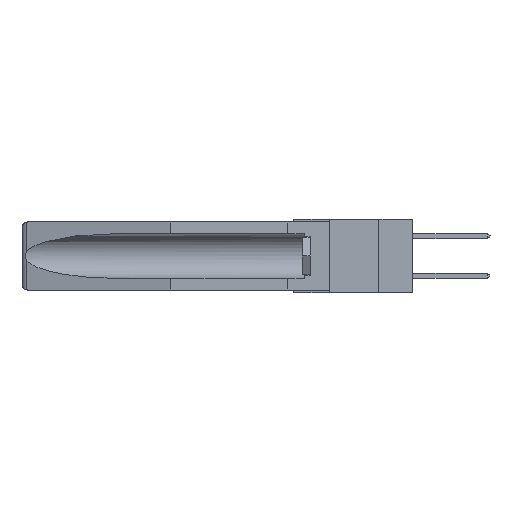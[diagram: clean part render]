
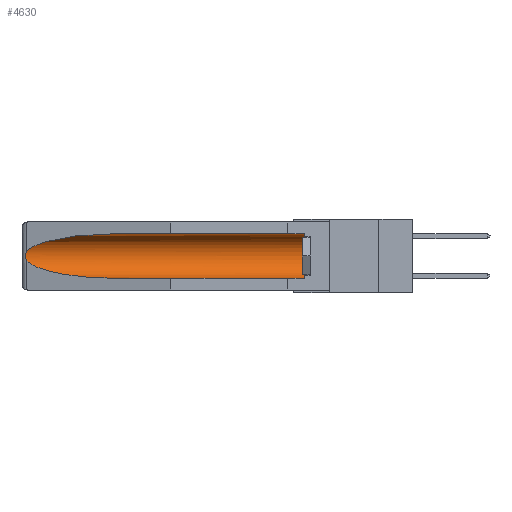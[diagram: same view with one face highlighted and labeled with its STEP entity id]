
A CAD part, left-side view. The second image highlights one B-rep face of the part: STEP entity #4630.
In plain terms, the highlighted cylindrical face has radius 2.857 mm (diameter 5.715 mm), a partial arc.
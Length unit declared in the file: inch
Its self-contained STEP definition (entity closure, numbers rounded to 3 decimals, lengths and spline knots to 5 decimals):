
#781 = CARTESIAN_POINT ( 'NONE',  ( 0.155, 1.07973, -0.284 ) ) ;
#1403 = CIRCLE ( 'NONE', #14783, 0.1125 ) ;
#1441 = CARTESIAN_POINT ( 'NONE',  ( 0.155, 0.126, -0.284 ) ) ;
#1802 = ORIENTED_EDGE ( 'NONE', *, *, #2086, .T. ) ;
#1818 = FACE_OUTER_BOUND ( 'NONE', #15287, .T. ) ;
#2026 = CARTESIAN_POINT ( 'NONE',  ( 0.155, -0.30754, -0.284 ) ) ;
#2086 = EDGE_CURVE ( 'NONE', #15935, #18991, #5848, .T. ) ;
#2349 = CARTESIAN_POINT ( 'NONE',  ( 0.2675, 1.53308, -0.17534 ) ) ;
#2480 = EDGE_CURVE ( 'NONE', #6593, #8802, #5024, .T. ) ;
#2681 = AXIS2_PLACEMENT_3D ( 'NONE', #6621, #21025, #12942 ) ;
#3083 = ORIENTED_EDGE ( 'NONE', *, *, #21367, .T. ) ;
#3285 = EDGE_CURVE ( 'NONE', #18991, #6593, #23365, .T. ) ;
#4249 = CARTESIAN_POINT ( 'NONE',  ( 0.21114, 1.30732, -0.059 ) ) ;
#4428 = CARTESIAN_POINT ( 'NONE',  ( 0.26655, 1.53094, -0.18657 ) ) ;
#4630 = ADVANCED_FACE ( 'NONE', ( #1818 ), #6944, .F. ) ;
#5024 =( BOUNDED_CURVE ( )  B_SPLINE_CURVE ( 3, ( #20943, #14566, #23131, #14912 ),
 .UNSPECIFIED., .F., .F. ) 
 B_SPLINE_CURVE_WITH_KNOTS ( ( 4, 4 ),
 ( 0.1948, 1.5708 ),
 .UNSPECIFIED. ) 
 CURVE ( )  GEOMETRIC_REPRESENTATION_ITEM ( )  RATIONAL_B_SPLINE_CURVE ( ( 1., 0.848, 0.848, 1. ) ) 
 REPRESENTATION_ITEM ( '' )  );
#5039 = VECTOR ( 'NONE', #22650, 39.37008 ) ;
#5651 = CARTESIAN_POINT ( 'NONE',  ( 0.155, 0.126, -0.1715 ) ) ;
#5848 =( BOUNDED_CURVE ( )  B_SPLINE_CURVE ( 3, ( #14773, #4249, #22893, #10552 ),
 .UNSPECIFIED., .F., .F. ) 
 B_SPLINE_CURVE_WITH_KNOTS ( ( 4, 4 ),
 ( 4.71239, 6.08839 ),
 .UNSPECIFIED. ) 
 CURVE ( )  GEOMETRIC_REPRESENTATION_ITEM ( )  RATIONAL_B_SPLINE_CURVE ( ( 1., 0.848, 0.848, 1. ) ) 
 REPRESENTATION_ITEM ( '' )  );
#6593 = VERTEX_POINT ( 'NONE', #18163 ) ;
#6621 = CARTESIAN_POINT ( 'NONE',  ( 0.155, -0.30754, -0.1715 ) ) ;
#6911 = CARTESIAN_POINT ( 'NONE',  ( 0.26597, 1.5296, -0.19026 ) ) ;
#6944 = CYLINDRICAL_SURFACE ( 'NONE', #2681, 0.1125 ) ;
#7244 = EDGE_CURVE ( 'NONE', #12657, #8291, #1403, .T. ) ;
#7865 = DIRECTION ( 'NONE',  ( 0., 1., 0. ) ) ;
#8291 = VERTEX_POINT ( 'NONE', #25321 ) ;
#8388 = CARTESIAN_POINT ( 'NONE',  ( 0.26654, 1.53092, -0.15636 ) ) ;
#8802 = VERTEX_POINT ( 'NONE', #781 ) ;
#9740 = CARTESIAN_POINT ( 'NONE',  ( 0.26537, 1.52718, -0.14972 ) ) ;
#10552 = CARTESIAN_POINT ( 'NONE',  ( 0.26537, 1.52718, -0.14972 ) ) ;
#10782 = ORIENTED_EDGE ( 'NONE', *, *, #7244, .T. ) ;
#10921 = ORIENTED_EDGE ( 'NONE', *, *, #3285, .T. ) ;
#12608 = CARTESIAN_POINT ( 'NONE',  ( 0.26597, 1.52961, -0.15275 ) ) ;
#12657 = VERTEX_POINT ( 'NONE', #1441 ) ;
#12786 = CARTESIAN_POINT ( 'NONE',  ( 0.2675, 1.53308, -0.16763 ) ) ;
#12942 = DIRECTION ( 'NONE',  ( 0., 0., 1. ) ) ;
#13358 = EDGE_CURVE ( 'NONE', #12657, #8802, #20469, .T. ) ;
#13946 = ORIENTED_EDGE ( 'NONE', *, *, #2480, .T. ) ;
#14011 = CARTESIAN_POINT ( 'NONE',  ( 0.155, -0.30754, -0.059 ) ) ;
#14087 = ORIENTED_EDGE ( 'NONE', *, *, #13358, .F. ) ;
#14566 = CARTESIAN_POINT ( 'NONE',  ( 0.25451, 1.48313, -0.24835 ) ) ;
#14665 = CARTESIAN_POINT ( 'NONE',  ( 0.2673, 1.5327, -0.16383 ) ) ;
#14773 = CARTESIAN_POINT ( 'NONE',  ( 0.155, 1.07973, -0.059 ) ) ;
#14783 = AXIS2_PLACEMENT_3D ( 'NONE', #5651, #15958, #20114 ) ;
#14912 = CARTESIAN_POINT ( 'NONE',  ( 0.155, 1.07973, -0.284 ) ) ;
#15287 = EDGE_LOOP ( 'NONE', ( #1802, #10921, #13946, #14087, #10782, #3083 ) ) ;
#15935 = VERTEX_POINT ( 'NONE', #25031 ) ;
#15958 = DIRECTION ( 'NONE',  ( 0., -1., 0. ) ) ;
#16729 = CARTESIAN_POINT ( 'NONE',  ( 0.2673, 1.53269, -0.17917 ) ) ;
#18163 = CARTESIAN_POINT ( 'NONE',  ( 0.26537, 1.52718, -0.19328 ) ) ;
#18991 = VERTEX_POINT ( 'NONE', #9740 ) ;
#20114 = DIRECTION ( 'NONE',  ( 0., 0., 1. ) ) ;
#20469 = LINE ( 'NONE', #2026, #5039 ) ;
#20943 = CARTESIAN_POINT ( 'NONE',  ( 0.26537, 1.52718, -0.19328 ) ) ;
#21025 = DIRECTION ( 'NONE',  ( 0., 1., 0. ) ) ;
#21223 = LINE ( 'NONE', #14011, #22239 ) ;
#21367 = EDGE_CURVE ( 'NONE', #8291, #15935, #21223, .T. ) ;
#22239 = VECTOR ( 'NONE', #7865, 39.37008 ) ;
#22650 = DIRECTION ( 'NONE',  ( 0., 1., 0. ) ) ;
#22893 = CARTESIAN_POINT ( 'NONE',  ( 0.25451, 1.48313, -0.09465 ) ) ;
#23131 = CARTESIAN_POINT ( 'NONE',  ( 0.21114, 1.30732, -0.284 ) ) ;
#23156 = CARTESIAN_POINT ( 'NONE',  ( 0.26537, 1.52718, -0.14972 ) ) ;
#23365 = B_SPLINE_CURVE_WITH_KNOTS ( 'NONE', 3,
 ( #23156, #12608, #8388, #14665, #12786, #2349, #16729, #4428, #6911, #23436 ),
 .UNSPECIFIED., .F., .F.,
 ( 4, 2, 2, 2, 4 ),
 ( 0., 0.00029, 0.00058, 0.00087, 0.00117 ),
 .UNSPECIFIED. ) ;
#23436 = CARTESIAN_POINT ( 'NONE',  ( 0.26537, 1.52718, -0.19328 ) ) ;
#25031 = CARTESIAN_POINT ( 'NONE',  ( 0.155, 1.07973, -0.059 ) ) ;
#25321 = CARTESIAN_POINT ( 'NONE',  ( 0.155, 0.126, -0.059 ) ) ;
